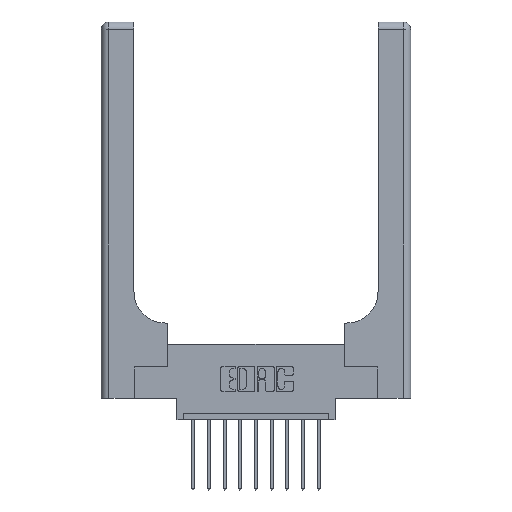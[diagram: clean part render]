
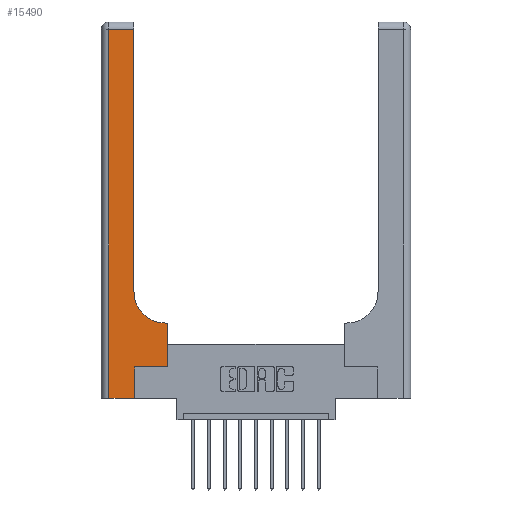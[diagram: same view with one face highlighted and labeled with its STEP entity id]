
A CAD part, top view. The second image highlights one B-rep face of the part: STEP entity #15490.
In plain terms, the highlighted planar face has unit normal (0, 0, 1).
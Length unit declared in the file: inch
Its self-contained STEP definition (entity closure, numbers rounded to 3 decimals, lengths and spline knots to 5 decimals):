
#1124 = CARTESIAN_POINT ( 'NONE',  ( 0.06, 3., 0.37 ) ) ;
#1229 = EDGE_CURVE ( 'NONE', #1948, #4448, #6611, .T. ) ;
#1266 = CARTESIAN_POINT ( 'NONE',  ( 0., 0., 0.37 ) ) ;
#1407 = CARTESIAN_POINT ( 'NONE',  ( 0.26, 3., 0.37 ) ) ;
#1487 = PLANE ( 'NONE',  #12366 ) ;
#1720 = CARTESIAN_POINT ( 'NONE',  ( 0.51, 0.6, 0.37 ) ) ;
#1948 = VERTEX_POINT ( 'NONE', #5506 ) ;
#2160 = EDGE_CURVE ( 'NONE', #7761, #9312, #12238, .T. ) ;
#2459 = EDGE_CURVE ( 'NONE', #6789, #1948, #4529, .T. ) ;
#2495 = CARTESIAN_POINT ( 'NONE',  ( 0.528, 0.6, 0.37 ) ) ;
#2998 = DIRECTION ( 'NONE',  ( 0., 1., 0. ) ) ;
#3103 = CARTESIAN_POINT ( 'NONE',  ( 0.26, 2.94, 0.37 ) ) ;
#3428 = EDGE_CURVE ( 'NONE', #14353, #6789, #4653, .T. ) ;
#3865 = DIRECTION ( 'NONE',  ( 1., 0., 0. ) ) ;
#3934 = CARTESIAN_POINT ( 'NONE',  ( 0.26, 0.85, 0.37 ) ) ;
#4136 = LINE ( 'NONE', #11176, #4316 ) ;
#4316 = VECTOR ( 'NONE', #12559, 39.37008 ) ;
#4448 = VERTEX_POINT ( 'NONE', #2495 ) ;
#4529 = LINE ( 'NONE', #9409, #10939 ) ;
#4551 = VECTOR ( 'NONE', #12064, 39.37008 ) ;
#4653 = LINE ( 'NONE', #12181, #11723 ) ;
#4780 = ORIENTED_EDGE ( 'NONE', *, *, #9978, .T. ) ;
#4945 = DIRECTION ( 'NONE',  ( 0., -1., 0. ) ) ;
#5092 = FACE_OUTER_BOUND ( 'NONE', #9814, .T. ) ;
#5506 = CARTESIAN_POINT ( 'NONE',  ( 0.528, 0.25, 0.37 ) ) ;
#5639 = CARTESIAN_POINT ( 'NONE',  ( 0.51, 0.85, 0.37 ) ) ;
#5790 = CARTESIAN_POINT ( 'NONE',  ( 0.265, 0., 0.37 ) ) ;
#6155 = EDGE_CURVE ( 'NONE', #9312, #14353, #13581, .T. ) ;
#6223 = ORIENTED_EDGE ( 'NONE', *, *, #3428, .T. ) ;
#6487 = ORIENTED_EDGE ( 'NONE', *, *, #7514, .T. ) ;
#6578 = EDGE_CURVE ( 'NONE', #11870, #7761, #15318, .T. ) ;
#6583 = CARTESIAN_POINT ( 'NONE',  ( 0.265, 0.25, 0.37 ) ) ;
#6611 = LINE ( 'NONE', #8859, #10638 ) ;
#6629 = CIRCLE ( 'NONE', #10459, 0.25 ) ;
#6789 = VERTEX_POINT ( 'NONE', #6583 ) ;
#6839 = CARTESIAN_POINT ( 'NONE',  ( 0.06, 2.94, 0.37 ) ) ;
#6849 = VERTEX_POINT ( 'NONE', #3934 ) ;
#6999 = DIRECTION ( 'NONE',  ( -1., 0., 0. ) ) ;
#7129 = DIRECTION ( 'NONE',  ( 0., 1., 0. ) ) ;
#7482 = ORIENTED_EDGE ( 'NONE', *, *, #6155, .T. ) ;
#7514 = EDGE_CURVE ( 'NONE', #6849, #11870, #13489, .T. ) ;
#7653 = DIRECTION ( 'NONE',  ( 0., 0., -1. ) ) ;
#7761 = VERTEX_POINT ( 'NONE', #6839 ) ;
#7864 = VECTOR ( 'NONE', #6999, 39.37008 ) ;
#8455 = ORIENTED_EDGE ( 'NONE', *, *, #2160, .T. ) ;
#8779 = DIRECTION ( 'NONE',  ( -1., 0., 0. ) ) ;
#8859 = CARTESIAN_POINT ( 'NONE',  ( 0.528, 0.25, 0.37 ) ) ;
#9312 = VERTEX_POINT ( 'NONE', #12339 ) ;
#9409 = CARTESIAN_POINT ( 'NONE',  ( 0.265, 0.25, 0.37 ) ) ;
#9814 = EDGE_LOOP ( 'NONE', ( #6487, #10888, #8455, #7482, #6223, #10302, #10153, #4780, #13864 ) ) ;
#9978 = EDGE_CURVE ( 'NONE', #4448, #10611, #4136, .T. ) ;
#10153 = ORIENTED_EDGE ( 'NONE', *, *, #1229, .T. ) ;
#10273 = DIRECTION ( 'NONE',  ( 1., 0., 0. ) ) ;
#10302 = ORIENTED_EDGE ( 'NONE', *, *, #2459, .T. ) ;
#10459 = AXIS2_PLACEMENT_3D ( 'NONE', #5639, #12857, #10273 ) ;
#10588 = EDGE_CURVE ( 'NONE', #10611, #6849, #6629, .T. ) ;
#10611 = VERTEX_POINT ( 'NONE', #1720 ) ;
#10638 = VECTOR ( 'NONE', #2998, 39.37008 ) ;
#10888 = ORIENTED_EDGE ( 'NONE', *, *, #6578, .T. ) ;
#10939 = VECTOR ( 'NONE', #11904, 39.37008 ) ;
#11012 = CARTESIAN_POINT ( 'NONE',  ( 0., 3., 0.37 ) ) ;
#11176 = CARTESIAN_POINT ( 'NONE',  ( 0.26, 0.6, 0.37 ) ) ;
#11380 = VECTOR ( 'NONE', #4945, 39.37008 ) ;
#11723 = VECTOR ( 'NONE', #7129, 39.37008 ) ;
#11870 = VERTEX_POINT ( 'NONE', #3103 ) ;
#11904 = DIRECTION ( 'NONE',  ( 1., 0., 0. ) ) ;
#12064 = DIRECTION ( 'NONE',  ( 0., 1., 0. ) ) ;
#12181 = CARTESIAN_POINT ( 'NONE',  ( 0.265, 0., 0.37 ) ) ;
#12238 = LINE ( 'NONE', #1124, #11380 ) ;
#12339 = CARTESIAN_POINT ( 'NONE',  ( 0.06, 0., 0.37 ) ) ;
#12366 = AXIS2_PLACEMENT_3D ( 'NONE', #11012, #7653, #8779 ) ;
#12559 = DIRECTION ( 'NONE',  ( -1., 0., 0. ) ) ;
#12857 = DIRECTION ( 'NONE',  ( 0., 0., -1. ) ) ;
#13489 = LINE ( 'NONE', #1407, #4551 ) ;
#13581 = LINE ( 'NONE', #1266, #13991 ) ;
#13864 = ORIENTED_EDGE ( 'NONE', *, *, #10588, .T. ) ;
#13991 = VECTOR ( 'NONE', #3865, 39.37008 ) ;
#14284 = CARTESIAN_POINT ( 'NONE',  ( 0., 2.94, 0.37 ) ) ;
#14353 = VERTEX_POINT ( 'NONE', #5790 ) ;
#15318 = LINE ( 'NONE', #14284, #7864 ) ;
#15490 = ADVANCED_FACE ( 'NONE', ( #5092 ), #1487, .F. ) ;
